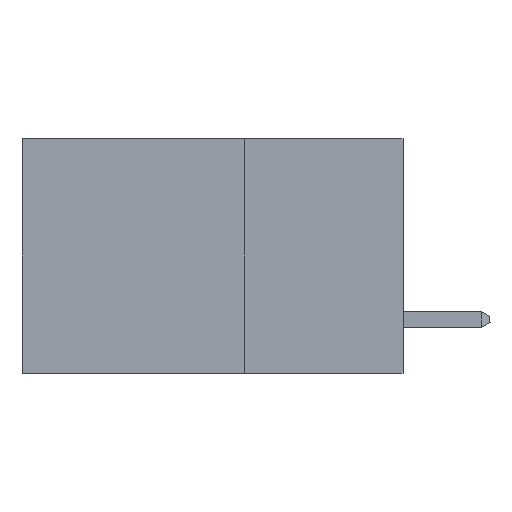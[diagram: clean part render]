
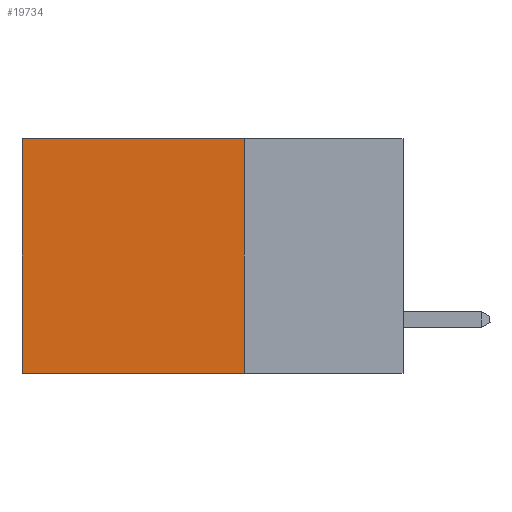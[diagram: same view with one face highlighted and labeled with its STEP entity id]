
A CAD part, left-side view. The second image highlights one B-rep face of the part: STEP entity #19734.
In plain terms, the highlighted planar face has unit normal (-1, 0, 0).
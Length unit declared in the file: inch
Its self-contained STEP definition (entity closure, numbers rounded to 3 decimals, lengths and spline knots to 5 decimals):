
#787 = ORIENTED_EDGE ( 'NONE', *, *, #2104, .F. ) ;
#1518 = DIRECTION ( 'NONE',  ( 0., 1., 0. ) ) ;
#2104 = EDGE_CURVE ( 'NONE', #6724, #14950, #4981, .T. ) ;
#2239 = ORIENTED_EDGE ( 'NONE', *, *, #17705, .T. ) ;
#2295 = EDGE_CURVE ( 'NONE', #3687, #9553, #10307, .T. ) ;
#2457 = ORIENTED_EDGE ( 'NONE', *, *, #7409, .F. ) ;
#3435 = CARTESIAN_POINT ( 'NONE',  ( 0.2875, 0.25, 0. ) ) ;
#3687 = VERTEX_POINT ( 'NONE', #10048 ) ;
#3800 = AXIS2_PLACEMENT_3D ( 'NONE', #5359, #3871, #16792 ) ;
#3871 = DIRECTION ( 'NONE',  ( 1., 0., 0. ) ) ;
#4142 = DIRECTION ( 'NONE',  ( 0., 0., -1. ) ) ;
#4202 = VECTOR ( 'NONE', #1518, 39.37008 ) ;
#4280 = FACE_OUTER_BOUND ( 'NONE', #7303, .T. ) ;
#4875 = LINE ( 'NONE', #13122, #20883 ) ;
#4937 = PLANE ( 'NONE',  #3800 ) ;
#4981 = LINE ( 'NONE', #16032, #4202 ) ;
#5359 = CARTESIAN_POINT ( 'NONE',  ( 0.2875, 0.25, 0. ) ) ;
#6500 = DIRECTION ( 'NONE',  ( 0., 1., 0. ) ) ;
#6724 = VERTEX_POINT ( 'NONE', #10192 ) ;
#7303 = EDGE_LOOP ( 'NONE', ( #2239, #787, #2457, #20807 ) ) ;
#7409 = EDGE_CURVE ( 'NONE', #3687, #6724, #10588, .T. ) ;
#8067 = DIRECTION ( 'NONE',  ( 0., 0., -1. ) ) ;
#8538 = VECTOR ( 'NONE', #6500, 39.37008 ) ;
#8734 = CARTESIAN_POINT ( 'NONE',  ( 0.2875, 0.6, 0. ) ) ;
#9020 = CARTESIAN_POINT ( 'NONE',  ( 0.2875, 0.25, 0. ) ) ;
#9097 = VECTOR ( 'NONE', #4142, 39.37008 ) ;
#9553 = VERTEX_POINT ( 'NONE', #8734 ) ;
#10048 = CARTESIAN_POINT ( 'NONE',  ( 0.2875, 0.25, 0. ) ) ;
#10192 = CARTESIAN_POINT ( 'NONE',  ( 0.2875, 0.25, -0.37 ) ) ;
#10307 = LINE ( 'NONE', #3435, #8538 ) ;
#10588 = LINE ( 'NONE', #9020, #9097 ) ;
#13122 = CARTESIAN_POINT ( 'NONE',  ( 0.2875, 0.6, 0. ) ) ;
#14950 = VERTEX_POINT ( 'NONE', #18110 ) ;
#16032 = CARTESIAN_POINT ( 'NONE',  ( 0.2875, 0.25, -0.37 ) ) ;
#16792 = DIRECTION ( 'NONE',  ( 0., 0., -1. ) ) ;
#17705 = EDGE_CURVE ( 'NONE', #9553, #14950, #4875, .T. ) ;
#18110 = CARTESIAN_POINT ( 'NONE',  ( 0.2875, 0.6, -0.37 ) ) ;
#19734 = ADVANCED_FACE ( 'NONE', ( #4280 ), #4937, .F. ) ;
#20807 = ORIENTED_EDGE ( 'NONE', *, *, #2295, .T. ) ;
#20883 = VECTOR ( 'NONE', #8067, 39.37008 ) ;
